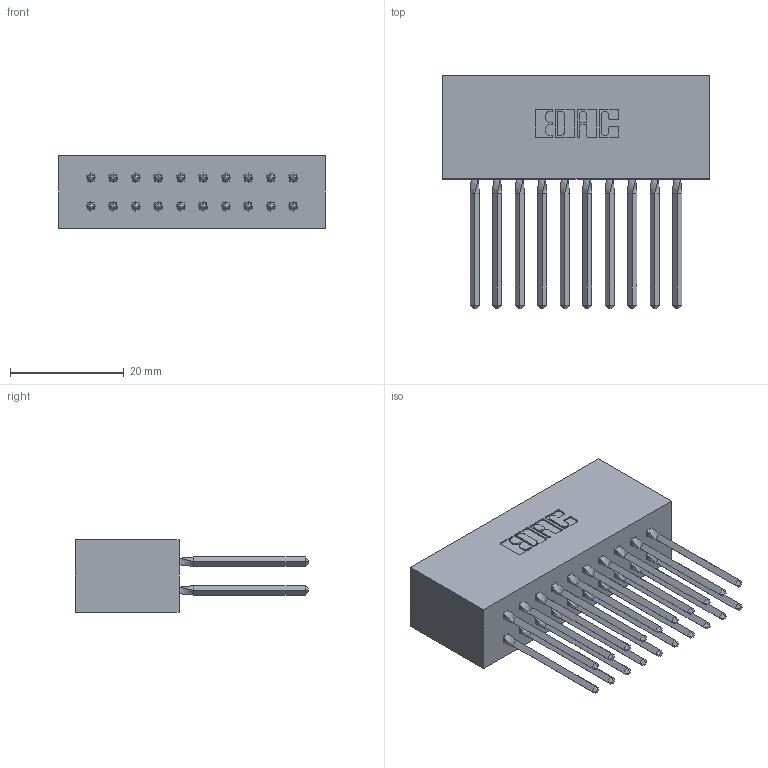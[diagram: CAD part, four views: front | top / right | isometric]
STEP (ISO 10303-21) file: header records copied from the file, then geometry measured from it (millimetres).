
FILE_DESCRIPTION (( 'STEP AP203' ), '1' );
FILE_NAME ('317-020-543-801.STEP', '2020-02-27T16:50:32', ( '' ), ( '' ), 'SwSTEP 2.0', 'SolidWorks 2016', '' );
FILE_SCHEMA (( 'CONFIG_CONTROL_DESIGN' ));
Length unit declared in the file: inch
Products named in the file (3): 317 Part_Lugless; 317-290-001_543; 317-020-543-801
Assembly tree (21 placements, depth 2):
  317-020-543-801
    317 Part_Lugless
    317-290-001_543  x20
Bounding box: 46.84 x 41.15 x 12.7 mm (x, y, z)
Volume: 8672 mm3; surface area: 12177 mm2
Topology: 21 solids, 21 shells, 1870 faces, 5179 edges, 3338 vertices
Faces by surface type: plane 1510, cylinder 280, bspline 80
Entity records: 18510 total; most frequent: CARTESIAN_POINT 3639, ORIENTED_EDGE 3138, DIRECTION 2615, EDGE_CURVE 1569, VECTOR 1321, LINE 1321, VERTEX_POINT 1039, AXIS2_PLACEMENT_3D 647
